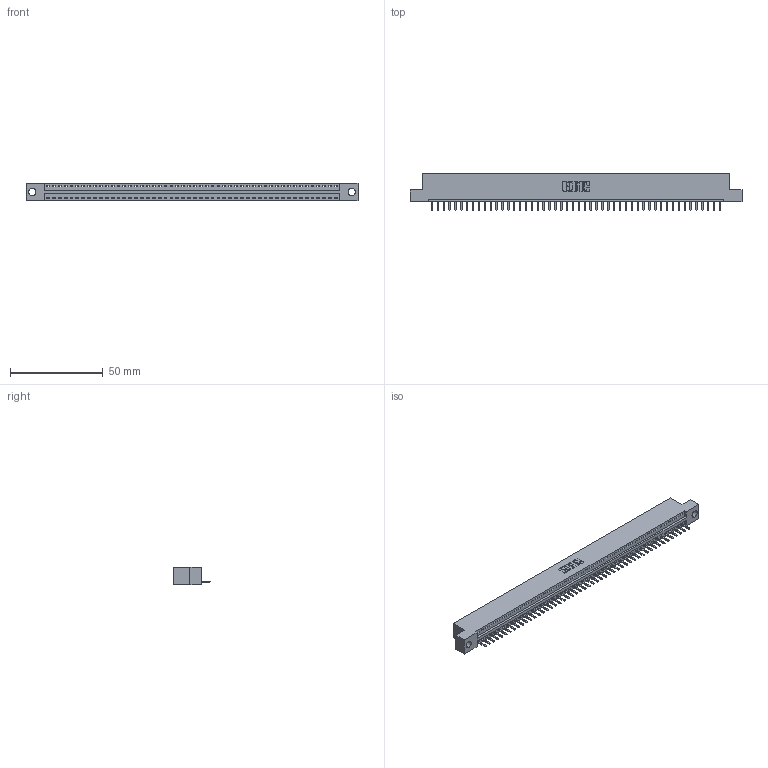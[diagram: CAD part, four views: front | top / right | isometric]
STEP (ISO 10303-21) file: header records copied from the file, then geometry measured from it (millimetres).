
FILE_DESCRIPTION (( 'STEP AP203' ), '1' );
FILE_NAME ('346-050-520-104.STEP', '2022-05-10T02:41:00', ( '' ), ( '' ), 'SwSTEP 2.0', 'SolidWorks 2020', '' );
FILE_SCHEMA (( 'CONFIG_CONTROL_DESIGN' ));
Length unit declared in the file: inch
Products named in the file (3): 346-050-520-104; 345-292-001_345-293-120; 346 Part_Flush Mounting Lugs - 0.156 Dia-TH
Assembly tree (51 placements, depth 2):
  346-050-520-104
    346 Part_Flush Mounting Lugs - 0.156 Dia-TH
    345-292-001_345-293-120  x50
Bounding box: 179.32 x 20.02 x 9.4 mm (x, y, z)
Volume: 16970.6 mm3; surface area: 20654.6 mm2
Topology: 51 solids, 51 shells, 3236 faces, 9565 edges, 6242 vertices
Faces by surface type: plane 2190, cylinder 1046
Entity records: 30487 total; most frequent: CARTESIAN_POINT 5244, ORIENTED_EDGE 5214, DIRECTION 4603, EDGE_CURVE 2607, LINE 2271, VECTOR 2271, VERTEX_POINT 1734, AXIS2_PLACEMENT_3D 1166
